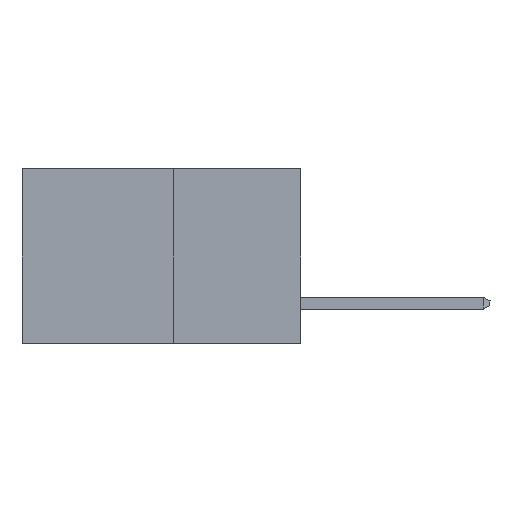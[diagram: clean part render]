
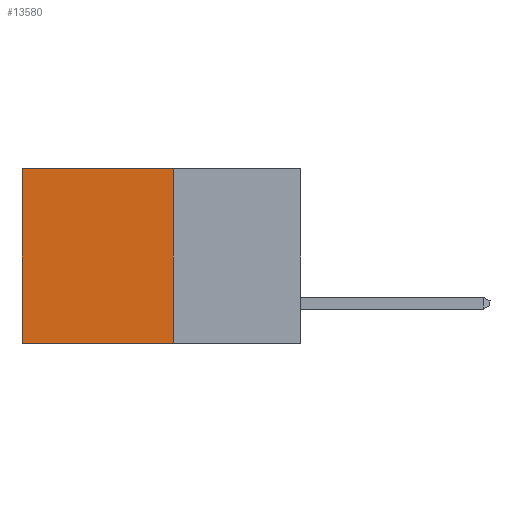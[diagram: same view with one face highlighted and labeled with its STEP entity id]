
A CAD part, left-side view. The second image highlights one B-rep face of the part: STEP entity #13580.
In plain terms, the highlighted planar face has unit normal (-1, 0, 0).
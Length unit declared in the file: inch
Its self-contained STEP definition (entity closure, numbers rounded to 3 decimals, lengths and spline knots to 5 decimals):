
#1013 = LINE ( 'NONE', #3683, #8029 ) ;
#1649 = VECTOR ( 'NONE', #13012, 39.37008 ) ;
#1977 = EDGE_CURVE ( 'NONE', #7242, #13838, #17292, .T. ) ;
#2312 = EDGE_CURVE ( 'NONE', #16091, #5292, #1013, .T. ) ;
#2576 = VECTOR ( 'NONE', #12128, 39.37008 ) ;
#3273 = CARTESIAN_POINT ( 'NONE',  ( 0.277, 0.27, 0. ) ) ;
#3683 = CARTESIAN_POINT ( 'NONE',  ( 0.277, 0.27, -0.37 ) ) ;
#4153 = EDGE_CURVE ( 'NONE', #5292, #13838, #6223, .T. ) ;
#4725 = CARTESIAN_POINT ( 'NONE',  ( 0.277, 0.59, 0. ) ) ;
#4773 = AXIS2_PLACEMENT_3D ( 'NONE', #15966, #17294, #9071 ) ;
#5292 = VERTEX_POINT ( 'NONE', #17137 ) ;
#5347 = LINE ( 'NONE', #3273, #1649 ) ;
#5771 = VECTOR ( 'NONE', #16949, 39.37008 ) ;
#5831 = ORIENTED_EDGE ( 'NONE', *, *, #1977, .T. ) ;
#6223 = LINE ( 'NONE', #16942, #5771 ) ;
#7242 = VERTEX_POINT ( 'NONE', #4725 ) ;
#8029 = VECTOR ( 'NONE', #12622, 39.37008 ) ;
#8460 = EDGE_LOOP ( 'NONE', ( #5831, #15866, #16535, #8920 ) ) ;
#8920 = ORIENTED_EDGE ( 'NONE', *, *, #17783, .T. ) ;
#9071 = DIRECTION ( 'NONE',  ( 0., 0., -1. ) ) ;
#12128 = DIRECTION ( 'NONE',  ( 0., 0., -1. ) ) ;
#12622 = DIRECTION ( 'NONE',  ( 0., 0., -1. ) ) ;
#13012 = DIRECTION ( 'NONE',  ( 0., 1., 0. ) ) ;
#13250 = CARTESIAN_POINT ( 'NONE',  ( 0.277, 0.27, 0. ) ) ;
#13580 = ADVANCED_FACE ( 'NONE', ( #17801 ), #14597, .F. ) ;
#13838 = VERTEX_POINT ( 'NONE', #15021 ) ;
#14482 = CARTESIAN_POINT ( 'NONE',  ( 0.277, 0.59, -0.37 ) ) ;
#14597 = PLANE ( 'NONE',  #4773 ) ;
#15021 = CARTESIAN_POINT ( 'NONE',  ( 0.277, 0.59, -0.37 ) ) ;
#15866 = ORIENTED_EDGE ( 'NONE', *, *, #4153, .F. ) ;
#15966 = CARTESIAN_POINT ( 'NONE',  ( 0.277, 0.27, -0.37 ) ) ;
#16091 = VERTEX_POINT ( 'NONE', #13250 ) ;
#16535 = ORIENTED_EDGE ( 'NONE', *, *, #2312, .F. ) ;
#16942 = CARTESIAN_POINT ( 'NONE',  ( 0.277, 0.27, -0.37 ) ) ;
#16949 = DIRECTION ( 'NONE',  ( 0., 1., 0. ) ) ;
#17137 = CARTESIAN_POINT ( 'NONE',  ( 0.277, 0.27, -0.37 ) ) ;
#17292 = LINE ( 'NONE', #14482, #2576 ) ;
#17294 = DIRECTION ( 'NONE',  ( 1., 0., 0. ) ) ;
#17783 = EDGE_CURVE ( 'NONE', #16091, #7242, #5347, .T. ) ;
#17801 = FACE_OUTER_BOUND ( 'NONE', #8460, .T. ) ;
